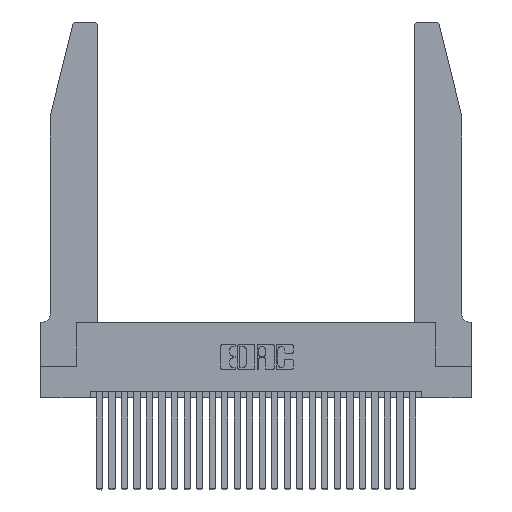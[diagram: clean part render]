
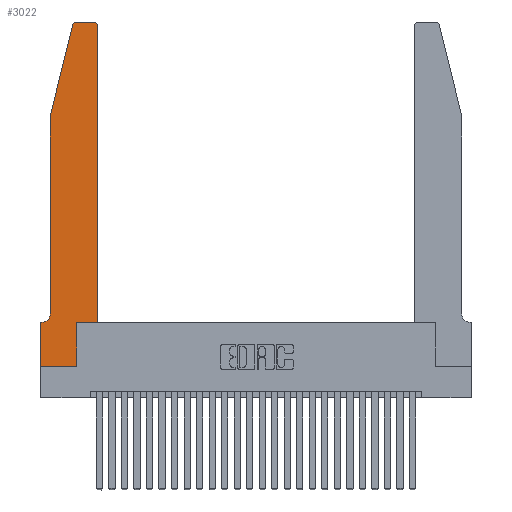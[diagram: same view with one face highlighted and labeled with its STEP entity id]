
A CAD part, top view. The second image highlights one B-rep face of the part: STEP entity #3022.
In plain terms, the highlighted planar face has unit normal (0, 0, 1).
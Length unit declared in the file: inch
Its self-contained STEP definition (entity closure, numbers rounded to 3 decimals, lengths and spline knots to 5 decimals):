
#204 = VERTEX_POINT ( 'NONE', #2064 ) ;
#367 = CARTESIAN_POINT ( 'NONE',  ( 0.4505, 2.72, 0.37 ) ) ;
#457 = LINE ( 'NONE', #25607, #27005 ) ;
#858 = VERTEX_POINT ( 'NONE', #4104 ) ;
#1097 = ORIENTED_EDGE ( 'NONE', *, *, #1144, .T. ) ;
#1144 = EDGE_CURVE ( 'NONE', #1342, #204, #17833, .T. ) ;
#1230 = VERTEX_POINT ( 'NONE', #17586 ) ;
#1342 = VERTEX_POINT ( 'NONE', #18237 ) ;
#1359 = CARTESIAN_POINT ( 'NONE',  ( 0., 0.35, 0.37 ) ) ;
#1548 = DIRECTION ( 'NONE',  ( 0., 0., 1. ) ) ;
#2064 = CARTESIAN_POINT ( 'NONE',  ( 0.4505, 0.35, 0.37 ) ) ;
#2132 = ORIENTED_EDGE ( 'NONE', *, *, #19155, .T. ) ;
#2229 = ORIENTED_EDGE ( 'NONE', *, *, #2646, .T. ) ;
#2293 = VECTOR ( 'NONE', #23494, 39.37008 ) ;
#2646 = EDGE_CURVE ( 'NONE', #13523, #8294, #22602, .T. ) ;
#2886 = FACE_OUTER_BOUND ( 'NONE', #23479, .T. ) ;
#2925 = VERTEX_POINT ( 'NONE', #7146 ) ;
#3022 = ADVANCED_FACE ( 'NONE', ( #2886 ), #26634, .T. ) ;
#3136 = ORIENTED_EDGE ( 'NONE', *, *, #17601, .T. ) ;
#3345 = CARTESIAN_POINT ( 'NONE',  ( 0.4505, 0.35, 0.37 ) ) ;
#3867 = VERTEX_POINT ( 'NONE', #10653 ) ;
#4104 = CARTESIAN_POINT ( 'NONE',  ( 0.25487, 2.72718, 0.37 ) ) ;
#4753 = DIRECTION ( 'NONE',  ( 0., 0., 1. ) ) ;
#4820 = DIRECTION ( 'NONE',  ( -1., 0., 0. ) ) ;
#4917 = LINE ( 'NONE', #23409, #2293 ) ;
#4998 = EDGE_CURVE ( 'NONE', #23740, #13523, #9347, .T. ) ;
#5873 = AXIS2_PLACEMENT_3D ( 'NONE', #10713, #4753, #13199 ) ;
#6255 = VERTEX_POINT ( 'NONE', #21344 ) ;
#6573 = CARTESIAN_POINT ( 'NONE',  ( 0.4505, 0.35, 0.37 ) ) ;
#7146 = CARTESIAN_POINT ( 'NONE',  ( 0.0055, 0.35, 0.37 ) ) ;
#7419 = EDGE_CURVE ( 'NONE', #8294, #1342, #21388, .T. ) ;
#7826 = ORIENTED_EDGE ( 'NONE', *, *, #7419, .T. ) ;
#8164 = ORIENTED_EDGE ( 'NONE', *, *, #18966, .T. ) ;
#8294 = VERTEX_POINT ( 'NONE', #24638 ) ;
#8340 = VECTOR ( 'NONE', #20427, 39.37008 ) ;
#8822 = CARTESIAN_POINT ( 'NONE',  ( 0.0755, 2., 0.37 ) ) ;
#9347 = LINE ( 'NONE', #23289, #20228 ) ;
#9547 = CIRCLE ( 'NONE', #24987, 0.07 ) ;
#9723 = CIRCLE ( 'NONE', #13714, 0.03 ) ;
#10629 = DIRECTION ( 'NONE',  ( 0., -1., 0. ) ) ;
#10653 = CARTESIAN_POINT ( 'NONE',  ( 0.4205, 2.75, 0.37 ) ) ;
#10713 = CARTESIAN_POINT ( 'NONE',  ( 0.284, 2.72, 0.37 ) ) ;
#11364 = ORIENTED_EDGE ( 'NONE', *, *, #17807, .T. ) ;
#11575 = ORIENTED_EDGE ( 'NONE', *, *, #21928, .T. ) ;
#11786 = CARTESIAN_POINT ( 'NONE',  ( 0.0755, 0.35, 0.37 ) ) ;
#11838 = EDGE_CURVE ( 'NONE', #6255, #2925, #9547, .T. ) ;
#12573 = CARTESIAN_POINT ( 'NONE',  ( 0., 0., 0.37 ) ) ;
#12776 = VECTOR ( 'NONE', #22348, 39.37008 ) ;
#13115 = DIRECTION ( 'NONE',  ( 1., 0., 0. ) ) ;
#13199 = DIRECTION ( 'NONE',  ( 1., 0., 0. ) ) ;
#13523 = VERTEX_POINT ( 'NONE', #17087 ) ;
#13714 = AXIS2_PLACEMENT_3D ( 'NONE', #18026, #22398, #26494 ) ;
#15186 = VECTOR ( 'NONE', #21279, 39.37008 ) ;
#15292 = CARTESIAN_POINT ( 'NONE',  ( 0.0755, 2., 0.37 ) ) ;
#15503 = AXIS2_PLACEMENT_3D ( 'NONE', #1359, #1548, #20455 ) ;
#15997 = VECTOR ( 'NONE', #25581, 39.37008 ) ;
#16347 = DIRECTION ( 'NONE',  ( 0., 1., 0. ) ) ;
#16492 = DIRECTION ( 'NONE',  ( 0., 0., -1. ) ) ;
#16666 = CARTESIAN_POINT ( 'NONE',  ( 0.0055, 0.42, 0.37 ) ) ;
#16698 = CARTESIAN_POINT ( 'NONE',  ( 0.2865, 0.35, 0.37 ) ) ;
#16769 = ORIENTED_EDGE ( 'NONE', *, *, #4998, .T. ) ;
#16885 = LINE ( 'NONE', #11786, #8340 ) ;
#17087 = CARTESIAN_POINT ( 'NONE',  ( 0., 0., 0.37 ) ) ;
#17586 = CARTESIAN_POINT ( 'NONE',  ( 0.284, 2.75, 0.37 ) ) ;
#17601 = EDGE_CURVE ( 'NONE', #21678, #6255, #27091, .T. ) ;
#17807 = EDGE_CURVE ( 'NONE', #23250, #3867, #9723, .T. ) ;
#17833 = LINE ( 'NONE', #6573, #15186 ) ;
#18026 = CARTESIAN_POINT ( 'NONE',  ( 0.4205, 2.72, 0.37 ) ) ;
#18237 = CARTESIAN_POINT ( 'NONE',  ( 0.2865, 0.35, 0.37 ) ) ;
#18966 = EDGE_CURVE ( 'NONE', #3867, #1230, #457, .T. ) ;
#19012 = VECTOR ( 'NONE', #13115, 39.37008 ) ;
#19155 = EDGE_CURVE ( 'NONE', #2925, #23740, #16885, .T. ) ;
#19403 = VECTOR ( 'NONE', #16347, 39.37008 ) ;
#19435 = ORIENTED_EDGE ( 'NONE', *, *, #11838, .T. ) ;
#20228 = VECTOR ( 'NONE', #10629, 39.37008 ) ;
#20342 = LINE ( 'NONE', #3345, #12776 ) ;
#20427 = DIRECTION ( 'NONE',  ( -1., 0., 0. ) ) ;
#20455 = DIRECTION ( 'NONE',  ( 1., 0., 0. ) ) ;
#21072 = DIRECTION ( 'NONE',  ( -1., 0., 0. ) ) ;
#21129 = ORIENTED_EDGE ( 'NONE', *, *, #26589, .T. ) ;
#21279 = DIRECTION ( 'NONE',  ( 1., 0., 0. ) ) ;
#21344 = CARTESIAN_POINT ( 'NONE',  ( 0.0755, 0.42, 0.37 ) ) ;
#21388 = LINE ( 'NONE', #16698, #19403 ) ;
#21678 = VERTEX_POINT ( 'NONE', #15292 ) ;
#21928 = EDGE_CURVE ( 'NONE', #204, #23250, #20342, .T. ) ;
#22288 = EDGE_CURVE ( 'NONE', #858, #21678, #4917, .T. ) ;
#22348 = DIRECTION ( 'NONE',  ( 0., 1., 0. ) ) ;
#22398 = DIRECTION ( 'NONE',  ( 0., 0., 1. ) ) ;
#22602 = LINE ( 'NONE', #12573, #19012 ) ;
#23250 = VERTEX_POINT ( 'NONE', #367 ) ;
#23289 = CARTESIAN_POINT ( 'NONE',  ( 0., 0., 0.37 ) ) ;
#23409 = CARTESIAN_POINT ( 'NONE',  ( 0.0755, 2., 0.37 ) ) ;
#23479 = EDGE_LOOP ( 'NONE', ( #8164, #21129, #23809, #3136, #19435, #2132, #16769, #2229, #7826, #1097, #11575, #11364 ) ) ;
#23494 = DIRECTION ( 'NONE',  ( -0.239, -0.971, 0. ) ) ;
#23740 = VERTEX_POINT ( 'NONE', #26920 ) ;
#23809 = ORIENTED_EDGE ( 'NONE', *, *, #22288, .T. ) ;
#24638 = CARTESIAN_POINT ( 'NONE',  ( 0.2865, 0., 0.37 ) ) ;
#24987 = AXIS2_PLACEMENT_3D ( 'NONE', #16666, #16492, #21072 ) ;
#25581 = DIRECTION ( 'NONE',  ( 0., -1., 0. ) ) ;
#25607 = CARTESIAN_POINT ( 'NONE',  ( 0.2605, 2.75, 0.37 ) ) ;
#26110 = CIRCLE ( 'NONE', #5873, 0.03 ) ;
#26494 = DIRECTION ( 'NONE',  ( 1., 0., 0. ) ) ;
#26589 = EDGE_CURVE ( 'NONE', #1230, #858, #26110, .T. ) ;
#26634 = PLANE ( 'NONE',  #15503 ) ;
#26920 = CARTESIAN_POINT ( 'NONE',  ( 0., 0.35, 0.37 ) ) ;
#27005 = VECTOR ( 'NONE', #4820, 39.37008 ) ;
#27091 = LINE ( 'NONE', #8822, #15997 ) ;
